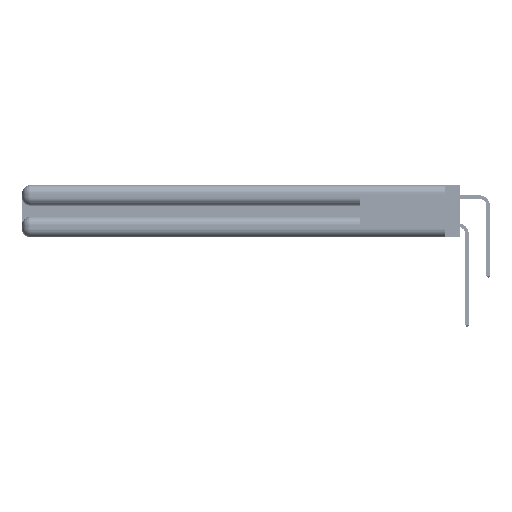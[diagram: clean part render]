
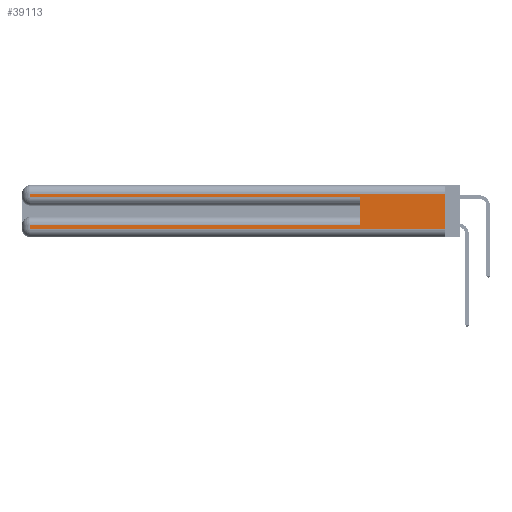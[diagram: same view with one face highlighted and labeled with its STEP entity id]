
A CAD part, left-side view. The second image highlights one B-rep face of the part: STEP entity #39113.
In plain terms, the highlighted planar face has unit normal (-1, 0, 0).
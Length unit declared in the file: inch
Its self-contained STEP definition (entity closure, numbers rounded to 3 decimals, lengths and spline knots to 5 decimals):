
#231 = CARTESIAN_POINT ( 'NONE',  ( 0., 0.6, 0.145 ) ) ;
#390 = ORIENTED_EDGE ( 'NONE', *, *, #19745, .T. ) ;
#477 = VERTEX_POINT ( 'NONE', #45309 ) ;
#1325 = DIRECTION ( 'NONE',  ( 0., -1., 0. ) ) ;
#3050 = ORIENTED_EDGE ( 'NONE', *, *, #39969, .T. ) ;
#3499 = CARTESIAN_POINT ( 'NONE',  ( 0., 2.94, 0.06 ) ) ;
#4872 = VECTOR ( 'NONE', #13413, 39.37008 ) ;
#6085 = CARTESIAN_POINT ( 'NONE',  ( 0., 2.94, 0.31 ) ) ;
#6379 = DIRECTION ( 'NONE',  ( 0., 0., -1. ) ) ;
#7953 = LINE ( 'NONE', #14788, #19366 ) ;
#8672 = VECTOR ( 'NONE', #33548, 39.37008 ) ;
#10919 = LINE ( 'NONE', #40968, #32301 ) ;
#13413 = DIRECTION ( 'NONE',  ( 0., -1., 0. ) ) ;
#13694 = CARTESIAN_POINT ( 'NONE',  ( 0., 0., 0.06 ) ) ;
#13876 = ORIENTED_EDGE ( 'NONE', *, *, #54459, .T. ) ;
#14595 = DIRECTION ( 'NONE',  ( 0., 0., -1. ) ) ;
#14788 = CARTESIAN_POINT ( 'NONE',  ( 0., 2.94, 0.37 ) ) ;
#14843 = VERTEX_POINT ( 'NONE', #35480 ) ;
#15309 = EDGE_CURVE ( 'NONE', #54022, #14843, #10919, .T. ) ;
#16362 = VECTOR ( 'NONE', #1325, 39.37008 ) ;
#16956 = PLANE ( 'NONE',  #19663 ) ;
#17638 = LINE ( 'NONE', #26332, #4872 ) ;
#18164 = ORIENTED_EDGE ( 'NONE', *, *, #15309, .T. ) ;
#18803 = VERTEX_POINT ( 'NONE', #42522 ) ;
#18969 = VERTEX_POINT ( 'NONE', #13694 ) ;
#19366 = VECTOR ( 'NONE', #6379, 39.37008 ) ;
#19663 = AXIS2_PLACEMENT_3D ( 'NONE', #25328, #21270, #50706 ) ;
#19745 = EDGE_CURVE ( 'NONE', #14843, #22615, #7953, .T. ) ;
#20728 = LINE ( 'NONE', #35336, #52971 ) ;
#21270 = DIRECTION ( 'NONE',  ( 1., 0., 0. ) ) ;
#21451 = LINE ( 'NONE', #24997, #8672 ) ;
#22615 = VERTEX_POINT ( 'NONE', #3499 ) ;
#24997 = CARTESIAN_POINT ( 'NONE',  ( 0., 0., 0.31 ) ) ;
#25263 = VERTEX_POINT ( 'NONE', #29118 ) ;
#25328 = CARTESIAN_POINT ( 'NONE',  ( 0., 0., 0.37 ) ) ;
#25546 = VERTEX_POINT ( 'NONE', #6085 ) ;
#25890 = DIRECTION ( 'NONE',  ( 0., 0., 1. ) ) ;
#26332 = CARTESIAN_POINT ( 'NONE',  ( 0., 0., 0.285 ) ) ;
#27311 = EDGE_CURVE ( 'NONE', #18803, #477, #17638, .T. ) ;
#29118 = CARTESIAN_POINT ( 'NONE',  ( 0., 0., 0.31 ) ) ;
#30745 = ORIENTED_EDGE ( 'NONE', *, *, #39361, .T. ) ;
#31240 = CARTESIAN_POINT ( 'NONE',  ( 0., 0., 0.06 ) ) ;
#32301 = VECTOR ( 'NONE', #32491, 39.37008 ) ;
#32491 = DIRECTION ( 'NONE',  ( 0., 1., 0. ) ) ;
#33089 = VECTOR ( 'NONE', #25890, 39.37008 ) ;
#33548 = DIRECTION ( 'NONE',  ( 0., 1., 0. ) ) ;
#33555 = ORIENTED_EDGE ( 'NONE', *, *, #49146, .F. ) ;
#33753 = ORIENTED_EDGE ( 'NONE', *, *, #27311, .T. ) ;
#35336 = CARTESIAN_POINT ( 'NONE',  ( 0., 0., 0.37 ) ) ;
#35480 = CARTESIAN_POINT ( 'NONE',  ( 0., 2.94, 0.085 ) ) ;
#39113 = ADVANCED_FACE ( 'NONE', ( #39630 ), #16956, .F. ) ;
#39361 = EDGE_CURVE ( 'NONE', #22615, #18969, #48747, .T. ) ;
#39523 = VECTOR ( 'NONE', #14595, 39.37008 ) ;
#39630 = FACE_OUTER_BOUND ( 'NONE', #46286, .T. ) ;
#39969 = EDGE_CURVE ( 'NONE', #25546, #18803, #50628, .T. ) ;
#40968 = CARTESIAN_POINT ( 'NONE',  ( 0., 0., 0.085 ) ) ;
#42522 = CARTESIAN_POINT ( 'NONE',  ( 0., 2.94, 0.285 ) ) ;
#42958 = LINE ( 'NONE', #231, #33089 ) ;
#43800 = DIRECTION ( 'NONE',  ( 0., 0., -1. ) ) ;
#45309 = CARTESIAN_POINT ( 'NONE',  ( 0., 0.6, 0.285 ) ) ;
#46286 = EDGE_LOOP ( 'NONE', ( #33555, #13876, #3050, #33753, #46909, #18164, #390, #30745 ) ) ;
#46909 = ORIENTED_EDGE ( 'NONE', *, *, #51374, .F. ) ;
#48103 = CARTESIAN_POINT ( 'NONE',  ( 0., 2.94, 0.37 ) ) ;
#48747 = LINE ( 'NONE', #31240, #16362 ) ;
#49146 = EDGE_CURVE ( 'NONE', #25263, #18969, #20728, .T. ) ;
#50628 = LINE ( 'NONE', #48103, #39523 ) ;
#50706 = DIRECTION ( 'NONE',  ( 0., 0., -1. ) ) ;
#50941 = CARTESIAN_POINT ( 'NONE',  ( 0., 0.6, 0.085 ) ) ;
#51374 = EDGE_CURVE ( 'NONE', #54022, #477, #42958, .T. ) ;
#52971 = VECTOR ( 'NONE', #43800, 39.37008 ) ;
#54022 = VERTEX_POINT ( 'NONE', #50941 ) ;
#54459 = EDGE_CURVE ( 'NONE', #25263, #25546, #21451, .T. ) ;
